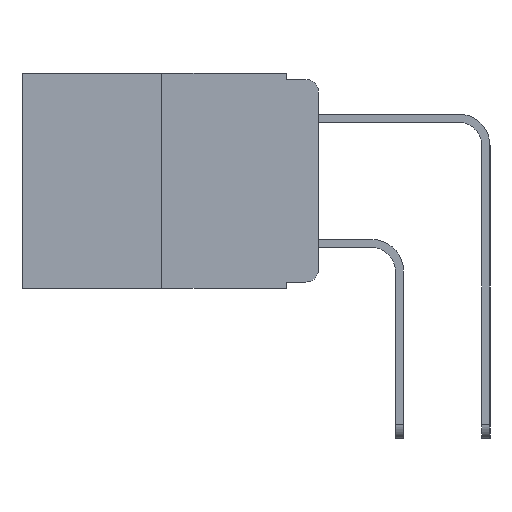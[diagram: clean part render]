
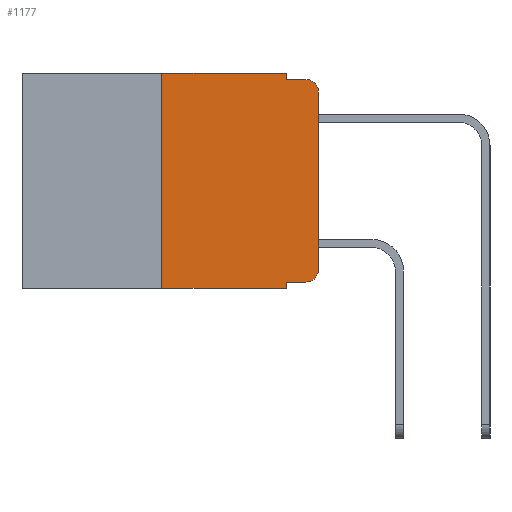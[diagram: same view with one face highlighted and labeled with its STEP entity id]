
A CAD part, left-side view. The second image highlights one B-rep face of the part: STEP entity #1177.
In plain terms, the highlighted planar face has unit normal (-1, 0, 0).
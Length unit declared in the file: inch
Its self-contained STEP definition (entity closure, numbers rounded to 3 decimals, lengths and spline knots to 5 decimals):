
#343 = EDGE_CURVE ( 'NONE', #7329, #2882, #1554, .T. ) ;
#668 = DIRECTION ( 'NONE',  ( 0., -1., 0. ) ) ;
#1156 = ORIENTED_EDGE ( 'NONE', *, *, #3886, .T. ) ;
#1177 = ADVANCED_FACE ( 'NONE', ( #14599 ), #6422, .F. ) ;
#1289 = EDGE_CURVE ( 'NONE', #6546, #13469, #10525, .T. ) ;
#1553 = DIRECTION ( 'NONE',  ( 0., 0., -1. ) ) ;
#1554 = LINE ( 'NONE', #9741, #3962 ) ;
#1602 = DIRECTION ( 'NONE',  ( -1., 0., 0. ) ) ;
#1646 = CARTESIAN_POINT ( 'NONE',  ( 0., 0.02, -0.03 ) ) ;
#1958 = VECTOR ( 'NONE', #6019, 39.37008 ) ;
#2261 = CARTESIAN_POINT ( 'NONE',  ( 0., 0.25, 0. ) ) ;
#2353 = EDGE_CURVE ( 'NONE', #2914, #7921, #3344, .T. ) ;
#2364 = VECTOR ( 'NONE', #4698, 39.37008 ) ;
#2882 = VERTEX_POINT ( 'NONE', #13446 ) ;
#2902 = VERTEX_POINT ( 'NONE', #2261 ) ;
#2914 = VERTEX_POINT ( 'NONE', #14712 ) ;
#2949 = VECTOR ( 'NONE', #3111, 39.37008 ) ;
#3111 = DIRECTION ( 'NONE',  ( 0., 0., 1. ) ) ;
#3137 = CARTESIAN_POINT ( 'NONE',  ( 0., 0.473, -0.343 ) ) ;
#3344 = CIRCLE ( 'NONE', #7652, 0.02 ) ;
#3422 = CARTESIAN_POINT ( 'NONE',  ( 0., 0.473, 0. ) ) ;
#3847 = VERTEX_POINT ( 'NONE', #13179 ) ;
#3886 = EDGE_CURVE ( 'NONE', #7921, #3847, #7248, .T. ) ;
#3962 = VECTOR ( 'NONE', #6172, 39.37008 ) ;
#4312 = VECTOR ( 'NONE', #668, 39.37008 ) ;
#4338 = EDGE_LOOP ( 'NONE', ( #1156, #9687, #14180, #11593, #9878, #10723, #11457, #12008, #13948, #14779 ) ) ;
#4586 = CARTESIAN_POINT ( 'NONE',  ( 0., 0.02, -0.313 ) ) ;
#4698 = DIRECTION ( 'NONE',  ( 0., -1., 0. ) ) ;
#4810 = DIRECTION ( 'NONE',  ( 0., 0., -1. ) ) ;
#4907 = CARTESIAN_POINT ( 'NONE',  ( 0., 0.051, 0. ) ) ;
#5736 = DIRECTION ( 'NONE',  ( 0., -1., 0. ) ) ;
#6019 = DIRECTION ( 'NONE',  ( 0., 0., -1. ) ) ;
#6172 = DIRECTION ( 'NONE',  ( 0., 0., -1. ) ) ;
#6188 = EDGE_CURVE ( 'NONE', #3847, #10622, #11603, .T. ) ;
#6422 = PLANE ( 'NONE',  #10440 ) ;
#6546 = VERTEX_POINT ( 'NONE', #8549 ) ;
#7248 = LINE ( 'NONE', #10193, #12776 ) ;
#7329 = VERTEX_POINT ( 'NONE', #7613 ) ;
#7613 = CARTESIAN_POINT ( 'NONE',  ( 0., 0.051, 0. ) ) ;
#7650 = LINE ( 'NONE', #3422, #10074 ) ;
#7652 = AXIS2_PLACEMENT_3D ( 'NONE', #4586, #8569, #7753 ) ;
#7753 = DIRECTION ( 'NONE',  ( 0., 0., -1. ) ) ;
#7921 = VERTEX_POINT ( 'NONE', #12220 ) ;
#8107 = CARTESIAN_POINT ( 'NONE',  ( 0., 0.051, -0.333 ) ) ;
#8276 = EDGE_CURVE ( 'NONE', #2882, #10622, #10805, .T. ) ;
#8549 = CARTESIAN_POINT ( 'NONE',  ( 0., 0.25, -0.343 ) ) ;
#8569 = DIRECTION ( 'NONE',  ( -1., 0., 0. ) ) ;
#8882 = EDGE_CURVE ( 'NONE', #10697, #2914, #14322, .T. ) ;
#9188 = CARTESIAN_POINT ( 'NONE',  ( 0., 0.473, 0. ) ) ;
#9286 = LINE ( 'NONE', #4907, #1958 ) ;
#9687 = ORIENTED_EDGE ( 'NONE', *, *, #6188, .T. ) ;
#9741 = CARTESIAN_POINT ( 'NONE',  ( 0., 0.051, 0. ) ) ;
#9802 = EDGE_CURVE ( 'NONE', #10697, #13469, #9286, .T. ) ;
#9832 = CARTESIAN_POINT ( 'NONE',  ( 0., 0.051, -0.343 ) ) ;
#9878 = ORIENTED_EDGE ( 'NONE', *, *, #12694, .F. ) ;
#9963 = CARTESIAN_POINT ( 'NONE',  ( 0., 0.051, -0.333 ) ) ;
#10074 = VECTOR ( 'NONE', #5736, 39.37008 ) ;
#10193 = CARTESIAN_POINT ( 'NONE',  ( 0., 0., 0. ) ) ;
#10257 = LINE ( 'NONE', #11307, #2949 ) ;
#10440 = AXIS2_PLACEMENT_3D ( 'NONE', #9188, #13576, #4810 ) ;
#10444 = VECTOR ( 'NONE', #11701, 39.37008 ) ;
#10525 = LINE ( 'NONE', #3137, #4312 ) ;
#10622 = VERTEX_POINT ( 'NONE', #11058 ) ;
#10697 = VERTEX_POINT ( 'NONE', #9963 ) ;
#10723 = ORIENTED_EDGE ( 'NONE', *, *, #12557, .F. ) ;
#10805 = LINE ( 'NONE', #15007, #10444 ) ;
#11058 = CARTESIAN_POINT ( 'NONE',  ( 0., 0.02, -0.01 ) ) ;
#11307 = CARTESIAN_POINT ( 'NONE',  ( 0., 0.25, 0. ) ) ;
#11457 = ORIENTED_EDGE ( 'NONE', *, *, #1289, .T. ) ;
#11593 = ORIENTED_EDGE ( 'NONE', *, *, #343, .F. ) ;
#11603 = CIRCLE ( 'NONE', #13265, 0.02 ) ;
#11701 = DIRECTION ( 'NONE',  ( 0., -1., 0. ) ) ;
#12008 = ORIENTED_EDGE ( 'NONE', *, *, #9802, .F. ) ;
#12220 = CARTESIAN_POINT ( 'NONE',  ( 0., 0., -0.313 ) ) ;
#12557 = EDGE_CURVE ( 'NONE', #6546, #2902, #10257, .T. ) ;
#12694 = EDGE_CURVE ( 'NONE', #2902, #7329, #7650, .T. ) ;
#12713 = DIRECTION ( 'NONE',  ( 0., 0., 1. ) ) ;
#12776 = VECTOR ( 'NONE', #12713, 39.37008 ) ;
#13179 = CARTESIAN_POINT ( 'NONE',  ( 0., 0., -0.03 ) ) ;
#13265 = AXIS2_PLACEMENT_3D ( 'NONE', #1646, #1602, #1553 ) ;
#13446 = CARTESIAN_POINT ( 'NONE',  ( 0., 0.051, -0.01 ) ) ;
#13469 = VERTEX_POINT ( 'NONE', #9832 ) ;
#13576 = DIRECTION ( 'NONE',  ( 1., 0., 0. ) ) ;
#13948 = ORIENTED_EDGE ( 'NONE', *, *, #8882, .T. ) ;
#14180 = ORIENTED_EDGE ( 'NONE', *, *, #8276, .F. ) ;
#14322 = LINE ( 'NONE', #8107, #2364 ) ;
#14599 = FACE_OUTER_BOUND ( 'NONE', #4338, .T. ) ;
#14712 = CARTESIAN_POINT ( 'NONE',  ( 0., 0.02, -0.333 ) ) ;
#14779 = ORIENTED_EDGE ( 'NONE', *, *, #2353, .T. ) ;
#15007 = CARTESIAN_POINT ( 'NONE',  ( 0., 0.051, -0.01 ) ) ;
